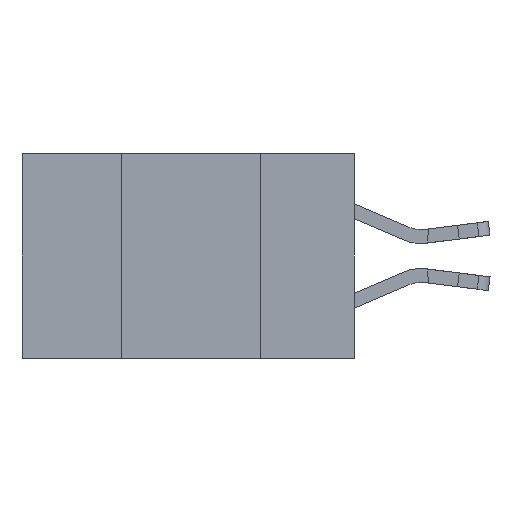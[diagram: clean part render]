
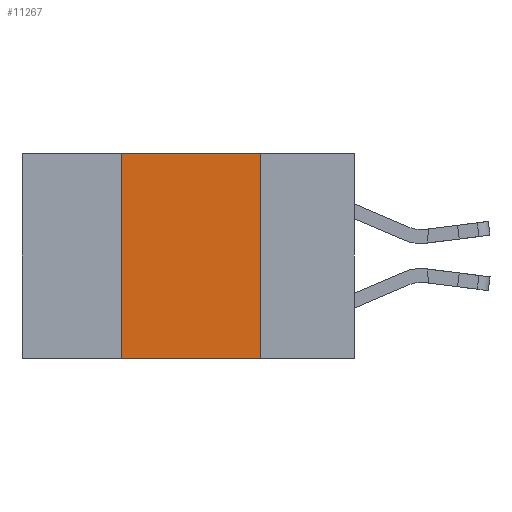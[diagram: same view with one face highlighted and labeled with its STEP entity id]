
A CAD part, left-side view. The second image highlights one B-rep face of the part: STEP entity #11267.
In plain terms, the highlighted planar face has unit normal (-1, 0, 0).
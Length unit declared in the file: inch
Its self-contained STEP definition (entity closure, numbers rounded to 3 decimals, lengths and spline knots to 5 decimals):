
#41 = VECTOR ( 'NONE', #14815, 39.37008 ) ;
#631 = CARTESIAN_POINT ( 'NONE',  ( 0., 0.17, -0.37 ) ) ;
#1063 = CARTESIAN_POINT ( 'NONE',  ( 0., 0.6, 0. ) ) ;
#2299 = VERTEX_POINT ( 'NONE', #5875 ) ;
#2549 = LINE ( 'NONE', #9517, #12199 ) ;
#3641 = LINE ( 'NONE', #631, #6375 ) ;
#3730 = DIRECTION ( 'NONE',  ( 0., 0., 1. ) ) ;
#3868 = CARTESIAN_POINT ( 'NONE',  ( 0., 0.42, -0.37 ) ) ;
#4142 = FACE_OUTER_BOUND ( 'NONE', #14164, .T. ) ;
#4375 = CARTESIAN_POINT ( 'NONE',  ( 0., 0.6, -0.37 ) ) ;
#4430 = LINE ( 'NONE', #3868, #11416 ) ;
#5424 = EDGE_CURVE ( 'NONE', #6482, #8484, #4430, .T. ) ;
#5875 = CARTESIAN_POINT ( 'NONE',  ( 0., 0.17, -0.37 ) ) ;
#6261 = ORIENTED_EDGE ( 'NONE', *, *, #13567, .F. ) ;
#6375 = VECTOR ( 'NONE', #12491, 39.37008 ) ;
#6482 = VERTEX_POINT ( 'NONE', #8696 ) ;
#7755 = DIRECTION ( 'NONE',  ( 0., 0., -1. ) ) ;
#8484 = VERTEX_POINT ( 'NONE', #14212 ) ;
#8696 = CARTESIAN_POINT ( 'NONE',  ( 0., 0.42, -0.37 ) ) ;
#8962 = VERTEX_POINT ( 'NONE', #10041 ) ;
#9433 = EDGE_CURVE ( 'NONE', #6482, #2299, #13984, .T. ) ;
#9517 = CARTESIAN_POINT ( 'NONE',  ( 0., 0.6, 0. ) ) ;
#9562 = AXIS2_PLACEMENT_3D ( 'NONE', #1063, #15484, #7755 ) ;
#10041 = CARTESIAN_POINT ( 'NONE',  ( 0., 0.17, 0. ) ) ;
#11267 = ADVANCED_FACE ( 'NONE', ( #4142 ), #12906, .F. ) ;
#11416 = VECTOR ( 'NONE', #3730, 39.37008 ) ;
#11582 = ORIENTED_EDGE ( 'NONE', *, *, #5424, .F. ) ;
#12193 = ORIENTED_EDGE ( 'NONE', *, *, #9433, .T. ) ;
#12199 = VECTOR ( 'NONE', #15942, 39.37008 ) ;
#12491 = DIRECTION ( 'NONE',  ( 0., 0., -1. ) ) ;
#12906 = PLANE ( 'NONE',  #9562 ) ;
#13567 = EDGE_CURVE ( 'NONE', #8962, #2299, #3641, .T. ) ;
#13984 = LINE ( 'NONE', #4375, #41 ) ;
#14164 = EDGE_LOOP ( 'NONE', ( #6261, #15727, #11582, #12193 ) ) ;
#14212 = CARTESIAN_POINT ( 'NONE',  ( 0., 0.42, 0. ) ) ;
#14815 = DIRECTION ( 'NONE',  ( 0., -1., 0. ) ) ;
#15484 = DIRECTION ( 'NONE',  ( 1., 0., 0. ) ) ;
#15727 = ORIENTED_EDGE ( 'NONE', *, *, #16561, .F. ) ;
#15942 = DIRECTION ( 'NONE',  ( 0., -1., 0. ) ) ;
#16561 = EDGE_CURVE ( 'NONE', #8484, #8962, #2549, .T. ) ;
